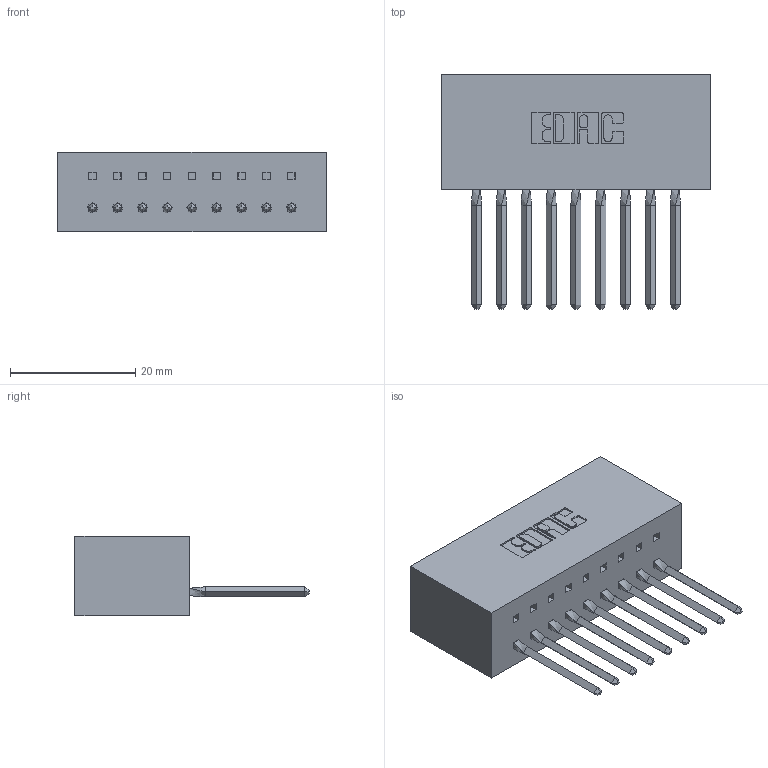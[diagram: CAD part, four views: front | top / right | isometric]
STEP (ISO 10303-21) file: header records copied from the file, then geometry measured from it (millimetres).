
FILE_DESCRIPTION (( 'STEP AP203' ), '1' );
FILE_NAME ('317-009-541-601.STEP', '2020-02-27T13:19:29', ( '' ), ( '' ), 'SwSTEP 2.0', 'SolidWorks 2016', '' );
FILE_SCHEMA (( 'CONFIG_CONTROL_DESIGN' ));
Length unit declared in the file: inch
Products named in the file (3): 317-009-541-601; 317 Part_Lugless; 317-290-002_541
Assembly tree (10 placements, depth 2):
  317-009-541-601
    317 Part_Lugless
    317-290-002_541  x9
Bounding box: 42.88 x 37.34 x 12.7 mm (x, y, z)
Volume: 7644 mm3; surface area: 9895 mm2
Topology: 10 solids, 10 shells, 1458 faces, 4145 edges, 2696 vertices
Faces by surface type: plane 1166, cylinder 256, bspline 36
Entity records: 18464 total; most frequent: CARTESIAN_POINT 3908, ORIENTED_EDGE 3170, DIRECTION 2571, EDGE_CURVE 1585, LINE 1229, VECTOR 1229, VERTEX_POINT 1048, AXIS2_PLACEMENT_3D 671
